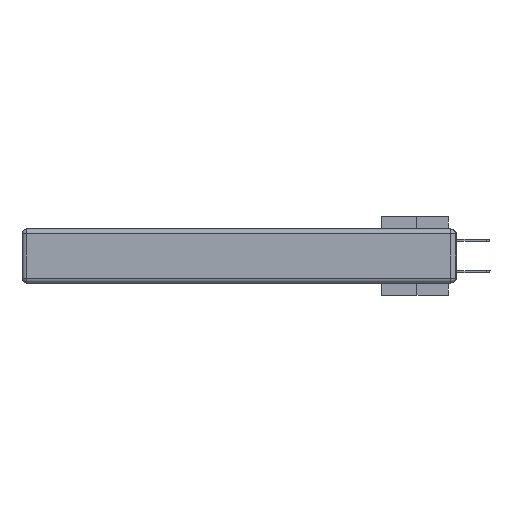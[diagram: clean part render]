
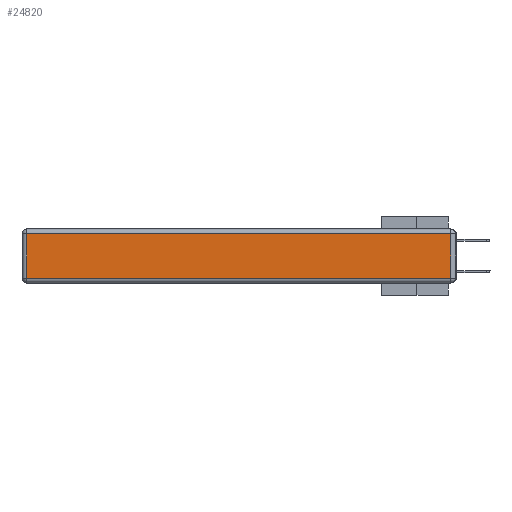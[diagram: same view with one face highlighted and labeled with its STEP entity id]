
A CAD part, left-side view. The second image highlights one B-rep face of the part: STEP entity #24820.
In plain terms, the highlighted planar face has unit normal (-1, 0, 0).
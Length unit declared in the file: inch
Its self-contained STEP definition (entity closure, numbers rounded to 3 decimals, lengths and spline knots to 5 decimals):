
#1117 = VECTOR ( 'NONE', #29927, 39.37008 ) ;
#1609 = VERTEX_POINT ( 'NONE', #1792 ) ;
#1768 = FACE_OUTER_BOUND ( 'NONE', #22799, .T. ) ;
#1792 = CARTESIAN_POINT ( 'NONE',  ( 0., 2.72, -0.313 ) ) ;
#2089 = DIRECTION ( 'NONE',  ( -1., 0., 0. ) ) ;
#4014 = ORIENTED_EDGE ( 'NONE', *, *, #5633, .T. ) ;
#4778 = DIRECTION ( 'NONE',  ( 0., 1., 0. ) ) ;
#5191 = EDGE_CURVE ( 'NONE', #16344, #1609, #17435, .T. ) ;
#5633 = EDGE_CURVE ( 'NONE', #17238, #16344, #27093, .T. ) ;
#5725 = ORIENTED_EDGE ( 'NONE', *, *, #6906, .T. ) ;
#6906 = EDGE_CURVE ( 'NONE', #1609, #16826, #7423, .T. ) ;
#7423 = LINE ( 'NONE', #22033, #14323 ) ;
#7555 = ORIENTED_EDGE ( 'NONE', *, *, #23535, .T. ) ;
#9068 = CARTESIAN_POINT ( 'NONE',  ( 0., 0.03, -0.313 ) ) ;
#9255 = CARTESIAN_POINT ( 'NONE',  ( 0., 2.72, -0.343 ) ) ;
#9468 = LINE ( 'NONE', #21619, #26326 ) ;
#11574 = CARTESIAN_POINT ( 'NONE',  ( 0., 2.72, -0.03 ) ) ;
#14323 = VECTOR ( 'NONE', #14990, 39.37008 ) ;
#14352 = AXIS2_PLACEMENT_3D ( 'NONE', #32119, #2089, #24732 ) ;
#14990 = DIRECTION ( 'NONE',  ( 0., -1., 0. ) ) ;
#16144 = ORIENTED_EDGE ( 'NONE', *, *, #5191, .T. ) ;
#16344 = VERTEX_POINT ( 'NONE', #11574 ) ;
#16826 = VERTEX_POINT ( 'NONE', #9068 ) ;
#17238 = VERTEX_POINT ( 'NONE', #28377 ) ;
#17239 = CARTESIAN_POINT ( 'NONE',  ( 0., 2.75, -0.03 ) ) ;
#17435 = LINE ( 'NONE', #9255, #1117 ) ;
#17914 = VECTOR ( 'NONE', #4778, 39.37008 ) ;
#21619 = CARTESIAN_POINT ( 'NONE',  ( 0., 0.03, -0.343 ) ) ;
#22033 = CARTESIAN_POINT ( 'NONE',  ( 0., 0., -0.313 ) ) ;
#22799 = EDGE_LOOP ( 'NONE', ( #5725, #7555, #4014, #16144 ) ) ;
#23535 = EDGE_CURVE ( 'NONE', #16826, #17238, #9468, .T. ) ;
#24575 = PLANE ( 'NONE',  #14352 ) ;
#24732 = DIRECTION ( 'NONE',  ( 0., 0., 1. ) ) ;
#24820 = ADVANCED_FACE ( 'NONE', ( #1768 ), #24575, .T. ) ;
#26326 = VECTOR ( 'NONE', #29014, 39.37008 ) ;
#27093 = LINE ( 'NONE', #17239, #17914 ) ;
#28377 = CARTESIAN_POINT ( 'NONE',  ( 0., 0.03, -0.03 ) ) ;
#29014 = DIRECTION ( 'NONE',  ( 0., 0., 1. ) ) ;
#29927 = DIRECTION ( 'NONE',  ( 0., 0., -1. ) ) ;
#32119 = CARTESIAN_POINT ( 'NONE',  ( 0., 0., -0.343 ) ) ;
